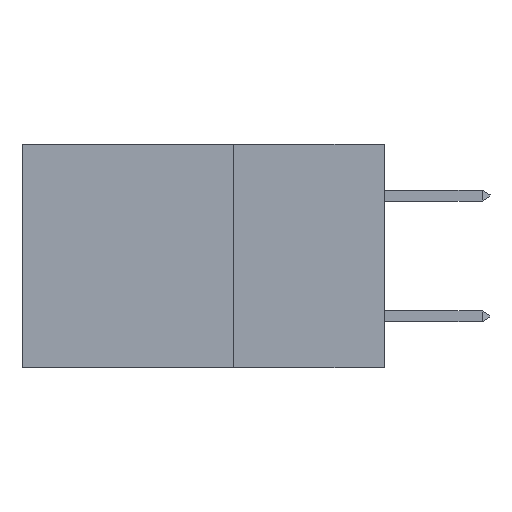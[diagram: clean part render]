
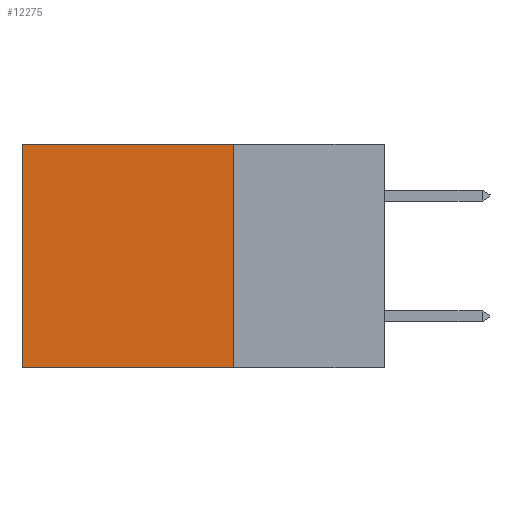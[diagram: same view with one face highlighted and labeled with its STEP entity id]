
A CAD part, left-side view. The second image highlights one B-rep face of the part: STEP entity #12275.
In plain terms, the highlighted planar face has unit normal (-1, 0, 0).
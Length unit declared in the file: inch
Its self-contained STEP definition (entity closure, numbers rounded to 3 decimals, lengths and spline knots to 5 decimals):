
#85 = DIRECTION ( 'NONE',  ( 0., 1., 0. ) ) ;
#553 = DIRECTION ( 'NONE',  ( 1., 0., 0. ) ) ;
#913 = VECTOR ( 'NONE', #85, 39.37008 ) ;
#1622 = VECTOR ( 'NONE', #12959, 39.37008 ) ;
#1986 = VERTEX_POINT ( 'NONE', #9971 ) ;
#1999 = DIRECTION ( 'NONE',  ( 0., 0., -1. ) ) ;
#3312 = EDGE_CURVE ( 'NONE', #10285, #6422, #6717, .T. ) ;
#4742 = CARTESIAN_POINT ( 'NONE',  ( 0.2875, 0.25, 0. ) ) ;
#6422 = VERTEX_POINT ( 'NONE', #20648 ) ;
#6717 = LINE ( 'NONE', #25679, #36199 ) ;
#7720 = AXIS2_PLACEMENT_3D ( 'NONE', #17575, #553, #34548 ) ;
#8507 = LINE ( 'NONE', #31467, #913 ) ;
#9815 = ORIENTED_EDGE ( 'NONE', *, *, #21477, .F. ) ;
#9971 = CARTESIAN_POINT ( 'NONE',  ( 0.2875, 0.25, -0.37 ) ) ;
#10285 = VERTEX_POINT ( 'NONE', #15741 ) ;
#11449 = VERTEX_POINT ( 'NONE', #16375 ) ;
#12275 = ADVANCED_FACE ( 'NONE', ( #17891 ), #14584, .F. ) ;
#12959 = DIRECTION ( 'NONE',  ( 0., 0., -1. ) ) ;
#14317 = ORIENTED_EDGE ( 'NONE', *, *, #3312, .T. ) ;
#14584 = PLANE ( 'NONE',  #7720 ) ;
#15741 = CARTESIAN_POINT ( 'NONE',  ( 0.2875, 0.25, 0. ) ) ;
#16303 = VECTOR ( 'NONE', #1999, 39.37008 ) ;
#16375 = CARTESIAN_POINT ( 'NONE',  ( 0.2875, 0.6, -0.37 ) ) ;
#16820 = LINE ( 'NONE', #30087, #1622 ) ;
#17575 = CARTESIAN_POINT ( 'NONE',  ( 0.2875, 0.25, 0. ) ) ;
#17891 = FACE_OUTER_BOUND ( 'NONE', #27300, .T. ) ;
#20043 = DIRECTION ( 'NONE',  ( 0., 1., 0. ) ) ;
#20244 = ORIENTED_EDGE ( 'NONE', *, *, #35536, .F. ) ;
#20648 = CARTESIAN_POINT ( 'NONE',  ( 0.2875, 0.6, 0. ) ) ;
#21477 = EDGE_CURVE ( 'NONE', #1986, #11449, #8507, .T. ) ;
#25679 = CARTESIAN_POINT ( 'NONE',  ( 0.2875, 0.25, 0. ) ) ;
#27300 = EDGE_LOOP ( 'NONE', ( #34291, #9815, #20244, #14317 ) ) ;
#29742 = EDGE_CURVE ( 'NONE', #6422, #11449, #16820, .T. ) ;
#30087 = CARTESIAN_POINT ( 'NONE',  ( 0.2875, 0.6, 0. ) ) ;
#31467 = CARTESIAN_POINT ( 'NONE',  ( 0.2875, 0.25, -0.37 ) ) ;
#31926 = LINE ( 'NONE', #4742, #16303 ) ;
#34291 = ORIENTED_EDGE ( 'NONE', *, *, #29742, .T. ) ;
#34548 = DIRECTION ( 'NONE',  ( 0., 0., -1. ) ) ;
#35536 = EDGE_CURVE ( 'NONE', #10285, #1986, #31926, .T. ) ;
#36199 = VECTOR ( 'NONE', #20043, 39.37008 ) ;
